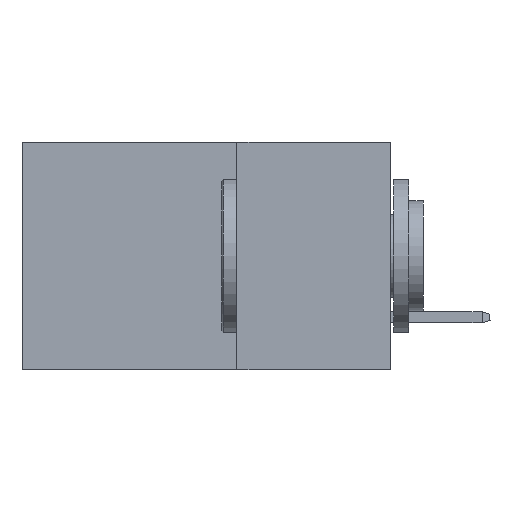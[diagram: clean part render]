
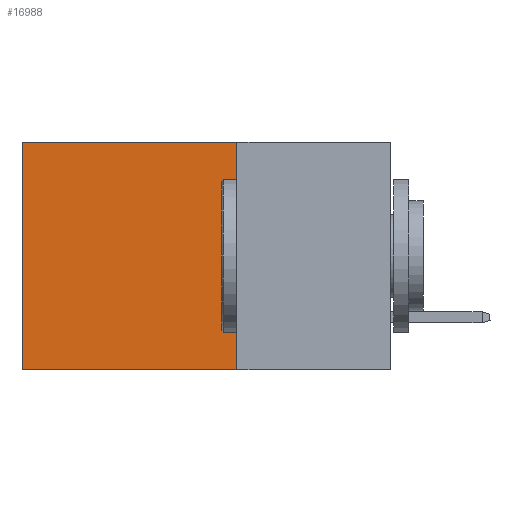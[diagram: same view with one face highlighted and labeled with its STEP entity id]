
A CAD part, left-side view. The second image highlights one B-rep face of the part: STEP entity #16988.
In plain terms, the highlighted planar face has unit normal (-1, 0, 0).
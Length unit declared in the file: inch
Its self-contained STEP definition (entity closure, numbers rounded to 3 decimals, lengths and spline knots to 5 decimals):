
#641 = AXIS2_PLACEMENT_3D ( 'NONE', #17176, #5616, #9509 ) ;
#2234 = CARTESIAN_POINT ( 'NONE',  ( 0.2875, 0.25, -0.37 ) ) ;
#2482 = VECTOR ( 'NONE', #20791, 39.37008 ) ;
#2904 = CARTESIAN_POINT ( 'NONE',  ( 0.2875, 0.25, 0. ) ) ;
#2926 = CARTESIAN_POINT ( 'NONE',  ( 0.2875, 0.6, 0. ) ) ;
#3255 = LINE ( 'NONE', #12587, #16210 ) ;
#4687 = CARTESIAN_POINT ( 'NONE',  ( 0.2875, 0.6, 0. ) ) ;
#5616 = DIRECTION ( 'NONE',  ( 1., 0., 0. ) ) ;
#5702 = VERTEX_POINT ( 'NONE', #17899 ) ;
#7131 = EDGE_CURVE ( 'NONE', #5702, #7758, #3255, .T. ) ;
#7670 = VERTEX_POINT ( 'NONE', #4687 ) ;
#7758 = VERTEX_POINT ( 'NONE', #2234 ) ;
#8070 = EDGE_CURVE ( 'NONE', #5702, #7670, #15005, .T. ) ;
#9509 = DIRECTION ( 'NONE',  ( 0., 0., -1. ) ) ;
#10026 = ORIENTED_EDGE ( 'NONE', *, *, #8070, .T. ) ;
#10440 = VECTOR ( 'NONE', #24128, 39.37008 ) ;
#11797 = PLANE ( 'NONE',  #641 ) ;
#12587 = CARTESIAN_POINT ( 'NONE',  ( 0.2875, 0.25, 0. ) ) ;
#12859 = FACE_OUTER_BOUND ( 'NONE', #17600, .T. ) ;
#13896 = LINE ( 'NONE', #2926, #16265 ) ;
#15005 = LINE ( 'NONE', #2904, #10440 ) ;
#16210 = VECTOR ( 'NONE', #19909, 39.37008 ) ;
#16265 = VECTOR ( 'NONE', #24650, 39.37008 ) ;
#16873 = ORIENTED_EDGE ( 'NONE', *, *, #24365, .F. ) ;
#16988 = ADVANCED_FACE ( 'NONE', ( #12859 ), #11797, .F. ) ;
#17176 = CARTESIAN_POINT ( 'NONE',  ( 0.2875, 0.25, 0. ) ) ;
#17600 = EDGE_LOOP ( 'NONE', ( #24111, #16873, #18222, #10026 ) ) ;
#17899 = CARTESIAN_POINT ( 'NONE',  ( 0.2875, 0.25, 0. ) ) ;
#18222 = ORIENTED_EDGE ( 'NONE', *, *, #7131, .F. ) ;
#18353 = CARTESIAN_POINT ( 'NONE',  ( 0.2875, 0.6, -0.37 ) ) ;
#19909 = DIRECTION ( 'NONE',  ( 0., 0., -1. ) ) ;
#20104 = EDGE_CURVE ( 'NONE', #7670, #21103, #13896, .T. ) ;
#20791 = DIRECTION ( 'NONE',  ( 0., 1., 0. ) ) ;
#21103 = VERTEX_POINT ( 'NONE', #18353 ) ;
#21195 = LINE ( 'NONE', #22478, #2482 ) ;
#22478 = CARTESIAN_POINT ( 'NONE',  ( 0.2875, 0.25, -0.37 ) ) ;
#24111 = ORIENTED_EDGE ( 'NONE', *, *, #20104, .T. ) ;
#24128 = DIRECTION ( 'NONE',  ( 0., 1., 0. ) ) ;
#24365 = EDGE_CURVE ( 'NONE', #7758, #21103, #21195, .T. ) ;
#24650 = DIRECTION ( 'NONE',  ( 0., 0., -1. ) ) ;
